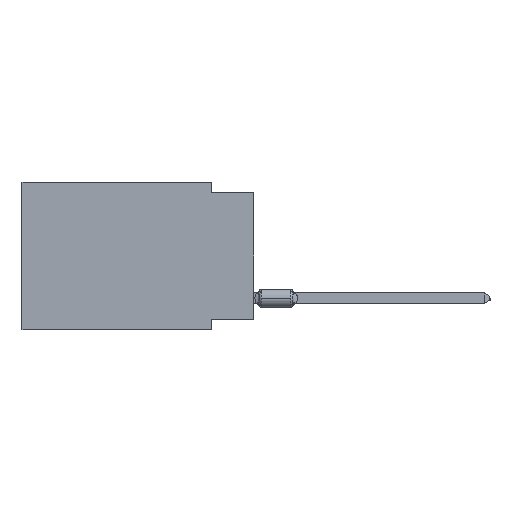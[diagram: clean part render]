
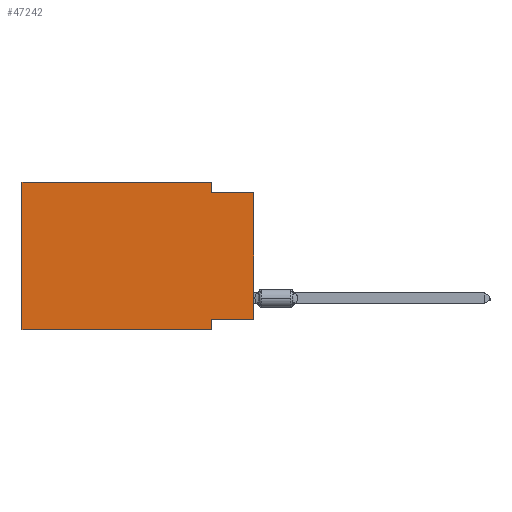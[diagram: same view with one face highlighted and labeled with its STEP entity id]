
A CAD part, left-side view. The second image highlights one B-rep face of the part: STEP entity #47242.
In plain terms, the highlighted planar face has unit normal (-1, 0, 0).
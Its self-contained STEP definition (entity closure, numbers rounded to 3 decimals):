
#297 = CARTESIAN_POINT ( 'NONE',  ( 0., 2.54, -8.89 ) ) ;
#330 = LINE ( 'NONE', #61741, #55079 ) ;
#859 = VECTOR ( 'NONE', #15912, 1000. ) ;
#1354 = LINE ( 'NONE', #22700, #27568 ) ;
#2640 = CARTESIAN_POINT ( 'NONE',  ( 0., 2.54, -8.255 ) ) ;
#4600 = LINE ( 'NONE', #50972, #859 ) ;
#4702 = CARTESIAN_POINT ( 'NONE',  ( 0., 2.54, 0. ) ) ;
#4883 = VERTEX_POINT ( 'NONE', #2640 ) ;
#6823 = CARTESIAN_POINT ( 'NONE',  ( 0., 0., -8.255 ) ) ;
#6876 = DIRECTION ( 'NONE',  ( 0., -1., 0. ) ) ;
#9215 = ORIENTED_EDGE ( 'NONE', *, *, #30644, .F. ) ;
#9227 = VECTOR ( 'NONE', #25363, 1000. ) ;
#9938 = EDGE_CURVE ( 'NONE', #18830, #27966, #4600, .T. ) ;
#10441 = LINE ( 'NONE', #65571, #18702 ) ;
#10956 = DIRECTION ( 'NONE',  ( 0., 0., -1. ) ) ;
#11336 = ORIENTED_EDGE ( 'NONE', *, *, #21279, .F. ) ;
#12618 = CARTESIAN_POINT ( 'NONE',  ( 0., 13.97, -8.89 ) ) ;
#15912 = DIRECTION ( 'NONE',  ( 0., -1., 0. ) ) ;
#16358 = ORIENTED_EDGE ( 'NONE', *, *, #39411, .F. ) ;
#16630 = EDGE_CURVE ( 'NONE', #24741, #46269, #21234, .T. ) ;
#18702 = VECTOR ( 'NONE', #44517, 1000. ) ;
#18830 = VERTEX_POINT ( 'NONE', #22476 ) ;
#19579 = EDGE_CURVE ( 'NONE', #41364, #46269, #330, .T. ) ;
#20088 = CARTESIAN_POINT ( 'NONE',  ( 0., 13.97, 0. ) ) ;
#20561 = AXIS2_PLACEMENT_3D ( 'NONE', #20088, #55836, #45147 ) ;
#20566 = VECTOR ( 'NONE', #6876, 1000. ) ;
#21234 = LINE ( 'NONE', #31582, #20566 ) ;
#21279 = EDGE_CURVE ( 'NONE', #64408, #18830, #1354, .T. ) ;
#22476 = CARTESIAN_POINT ( 'NONE',  ( 0., 13.97, 0. ) ) ;
#22700 = CARTESIAN_POINT ( 'NONE',  ( 0., 13.97, 0. ) ) ;
#22913 = CARTESIAN_POINT ( 'NONE',  ( 0., 0., -0.635 ) ) ;
#24741 = VERTEX_POINT ( 'NONE', #42063 ) ;
#25363 = DIRECTION ( 'NONE',  ( 0., 1., 0. ) ) ;
#27568 = VECTOR ( 'NONE', #52436, 1000. ) ;
#27966 = VERTEX_POINT ( 'NONE', #4702 ) ;
#30621 = EDGE_LOOP ( 'NONE', ( #56675, #43404, #16358, #43657, #11336, #45003, #9215, #42684 ) ) ;
#30644 = EDGE_CURVE ( 'NONE', #4883, #61782, #51678, .T. ) ;
#31582 = CARTESIAN_POINT ( 'NONE',  ( 0., 0., -0.635 ) ) ;
#34498 = PLANE ( 'NONE',  #20561 ) ;
#35092 = VECTOR ( 'NONE', #41628, 1000. ) ;
#37062 = EDGE_CURVE ( 'NONE', #64408, #61782, #10441, .T. ) ;
#39406 = CARTESIAN_POINT ( 'NONE',  ( 0., 0., -8.255 ) ) ;
#39411 = EDGE_CURVE ( 'NONE', #27966, #24741, #51329, .T. ) ;
#41237 = CARTESIAN_POINT ( 'NONE',  ( 0., 2.54, -8.89 ) ) ;
#41364 = VERTEX_POINT ( 'NONE', #6823 ) ;
#41628 = DIRECTION ( 'NONE',  ( 0., 0., -1. ) ) ;
#42063 = CARTESIAN_POINT ( 'NONE',  ( 0., 2.54, -0.635 ) ) ;
#42684 = ORIENTED_EDGE ( 'NONE', *, *, #52589, .F. ) ;
#43404 = ORIENTED_EDGE ( 'NONE', *, *, #16630, .F. ) ;
#43657 = ORIENTED_EDGE ( 'NONE', *, *, #9938, .F. ) ;
#44517 = DIRECTION ( 'NONE',  ( 0., -1., 0. ) ) ;
#45003 = ORIENTED_EDGE ( 'NONE', *, *, #37062, .T. ) ;
#45147 = DIRECTION ( 'NONE',  ( 0., 0., -1. ) ) ;
#45389 = LINE ( 'NONE', #39406, #9227 ) ;
#46269 = VERTEX_POINT ( 'NONE', #22913 ) ;
#47242 = ADVANCED_FACE ( 'NONE', ( #65536 ), #34498, .F. ) ;
#50892 = VECTOR ( 'NONE', #10956, 1000. ) ;
#50972 = CARTESIAN_POINT ( 'NONE',  ( 0., 13.97, 0. ) ) ;
#51329 = LINE ( 'NONE', #61354, #35092 ) ;
#51678 = LINE ( 'NONE', #297, #50892 ) ;
#52436 = DIRECTION ( 'NONE',  ( 0., 0., 1. ) ) ;
#52589 = EDGE_CURVE ( 'NONE', #41364, #4883, #45389, .T. ) ;
#55079 = VECTOR ( 'NONE', #63327, 1000. ) ;
#55836 = DIRECTION ( 'NONE',  ( 1., 0., 0. ) ) ;
#56675 = ORIENTED_EDGE ( 'NONE', *, *, #19579, .T. ) ;
#61354 = CARTESIAN_POINT ( 'NONE',  ( 0., 2.54, 0. ) ) ;
#61741 = CARTESIAN_POINT ( 'NONE',  ( 0., 0., 0. ) ) ;
#61782 = VERTEX_POINT ( 'NONE', #41237 ) ;
#63327 = DIRECTION ( 'NONE',  ( 0., 0., 1. ) ) ;
#64408 = VERTEX_POINT ( 'NONE', #12618 ) ;
#65536 = FACE_OUTER_BOUND ( 'NONE', #30621, .T. ) ;
#65571 = CARTESIAN_POINT ( 'NONE',  ( 0., 13.97, -8.89 ) ) ;
